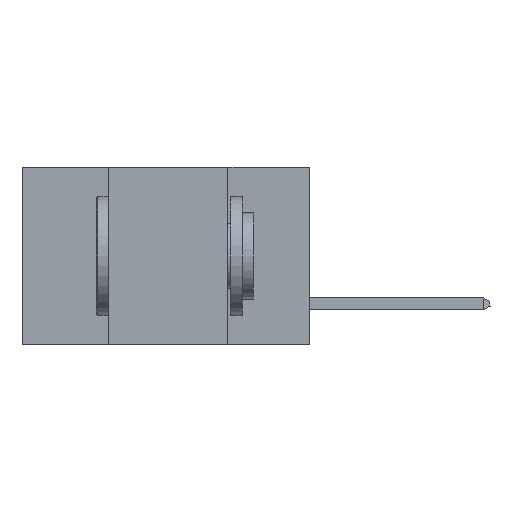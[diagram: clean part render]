
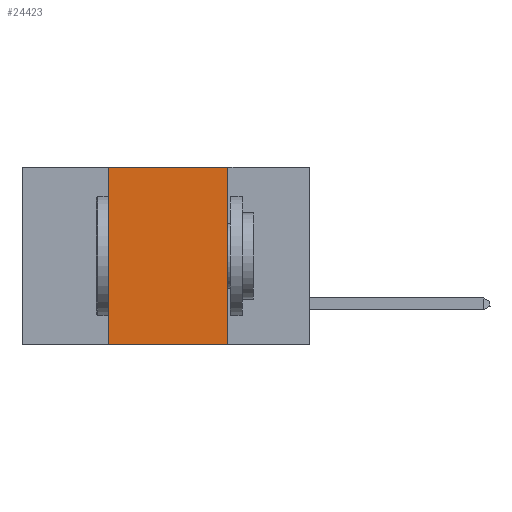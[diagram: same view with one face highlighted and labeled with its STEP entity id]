
A CAD part, left-side view. The second image highlights one B-rep face of the part: STEP entity #24423.
In plain terms, the highlighted planar face has unit normal (-1, 0, 0).
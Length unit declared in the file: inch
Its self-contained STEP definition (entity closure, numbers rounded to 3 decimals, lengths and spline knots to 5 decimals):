
#677 = EDGE_CURVE ( 'NONE', #24989, #2838, #17504, .T. ) ;
#2010 = LINE ( 'NONE', #39225, #37514 ) ;
#2379 = CARTESIAN_POINT ( 'NONE',  ( 0., 0.6, -0.37 ) ) ;
#2838 = VERTEX_POINT ( 'NONE', #8620 ) ;
#3004 = CARTESIAN_POINT ( 'NONE',  ( 0., 0.17, 0. ) ) ;
#4861 = VECTOR ( 'NONE', #46015, 39.37008 ) ;
#5060 = ORIENTED_EDGE ( 'NONE', *, *, #677, .F. ) ;
#5688 = CARTESIAN_POINT ( 'NONE',  ( 0., 0.6, 0. ) ) ;
#6154 = DIRECTION ( 'NONE',  ( 0., -1., 0. ) ) ;
#8620 = CARTESIAN_POINT ( 'NONE',  ( 0., 0.42, 0. ) ) ;
#9541 = DIRECTION ( 'NONE',  ( 0., -1., 0. ) ) ;
#9923 = EDGE_CURVE ( 'NONE', #24989, #19897, #11323, .T. ) ;
#9956 = PLANE ( 'NONE',  #28060 ) ;
#11323 = LINE ( 'NONE', #2379, #38816 ) ;
#17504 = LINE ( 'NONE', #42319, #4861 ) ;
#18859 = CARTESIAN_POINT ( 'NONE',  ( 0., 0.6, 0. ) ) ;
#19869 = LINE ( 'NONE', #5688, #24712 ) ;
#19897 = VERTEX_POINT ( 'NONE', #27808 ) ;
#20002 = FACE_OUTER_BOUND ( 'NONE', #46448, .T. ) ;
#23945 = DIRECTION ( 'NONE',  ( 0., 0., -1. ) ) ;
#24423 = ADVANCED_FACE ( 'NONE', ( #20002 ), #9956, .F. ) ;
#24712 = VECTOR ( 'NONE', #9541, 39.37008 ) ;
#24989 = VERTEX_POINT ( 'NONE', #25929 ) ;
#25769 = EDGE_CURVE ( 'NONE', #2838, #45788, #19869, .T. ) ;
#25929 = CARTESIAN_POINT ( 'NONE',  ( 0., 0.42, -0.37 ) ) ;
#26760 = DIRECTION ( 'NONE',  ( 1., 0., 0. ) ) ;
#27808 = CARTESIAN_POINT ( 'NONE',  ( 0., 0.17, -0.37 ) ) ;
#28060 = AXIS2_PLACEMENT_3D ( 'NONE', #18859, #26760, #42140 ) ;
#31422 = ORIENTED_EDGE ( 'NONE', *, *, #9923, .T. ) ;
#35145 = EDGE_CURVE ( 'NONE', #45788, #19897, #2010, .T. ) ;
#37113 = ORIENTED_EDGE ( 'NONE', *, *, #35145, .F. ) ;
#37514 = VECTOR ( 'NONE', #23945, 39.37008 ) ;
#38816 = VECTOR ( 'NONE', #6154, 39.37008 ) ;
#39225 = CARTESIAN_POINT ( 'NONE',  ( 0., 0.17, 0. ) ) ;
#42140 = DIRECTION ( 'NONE',  ( 0., 0., -1. ) ) ;
#42319 = CARTESIAN_POINT ( 'NONE',  ( 0., 0.42, 0. ) ) ;
#45788 = VERTEX_POINT ( 'NONE', #3004 ) ;
#46015 = DIRECTION ( 'NONE',  ( 0., 0., 1. ) ) ;
#46448 = EDGE_LOOP ( 'NONE', ( #37113, #48613, #5060, #31422 ) ) ;
#48613 = ORIENTED_EDGE ( 'NONE', *, *, #25769, .F. ) ;
